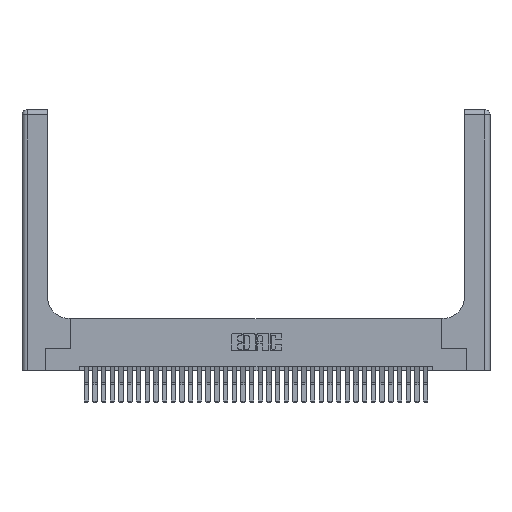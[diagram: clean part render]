
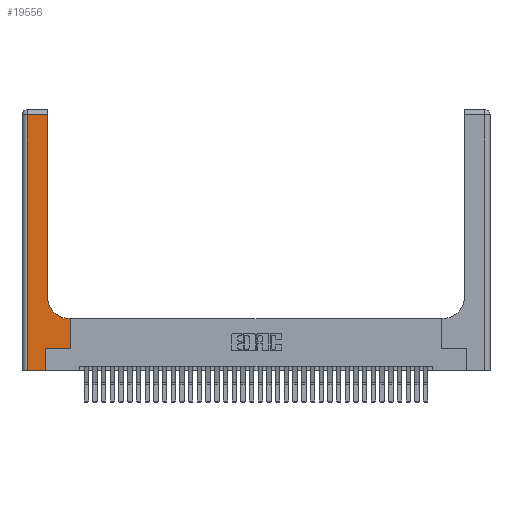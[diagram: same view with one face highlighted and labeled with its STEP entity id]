
A CAD part, top view. The second image highlights one B-rep face of the part: STEP entity #19556.
In plain terms, the highlighted planar face has unit normal (0, 0, 1).
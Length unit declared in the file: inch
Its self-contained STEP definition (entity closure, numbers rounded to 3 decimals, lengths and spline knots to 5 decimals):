
#221 = ORIENTED_EDGE ( 'NONE', *, *, #7504, .T. ) ;
#449 = DIRECTION ( 'NONE',  ( 1., 0., 0. ) ) ;
#683 = CARTESIAN_POINT ( 'NONE',  ( 0.5585, 0.25, 0.37 ) ) ;
#2005 = CARTESIAN_POINT ( 'NONE',  ( 0., 3., 0.37 ) ) ;
#2176 = ORIENTED_EDGE ( 'NONE', *, *, #9632, .T. ) ;
#2762 = CARTESIAN_POINT ( 'NONE',  ( 0., 2.94, 0.37 ) ) ;
#2857 = CARTESIAN_POINT ( 'NONE',  ( 0.2915, 0.6, 0.37 ) ) ;
#3098 = VECTOR ( 'NONE', #32187, 39.37008 ) ;
#3341 = EDGE_CURVE ( 'NONE', #21433, #3761, #20423, .T. ) ;
#3761 = VERTEX_POINT ( 'NONE', #10669 ) ;
#4089 = LINE ( 'NONE', #33217, #33562 ) ;
#4102 = CARTESIAN_POINT ( 'NONE',  ( 0.2915, 0.85, 0.37 ) ) ;
#4338 = VERTEX_POINT ( 'NONE', #13151 ) ;
#5379 = DIRECTION ( 'NONE',  ( 0., -1., 0. ) ) ;
#5756 = DIRECTION ( 'NONE',  ( -1., 0., 0. ) ) ;
#6155 = ORIENTED_EDGE ( 'NONE', *, *, #3341, .T. ) ;
#6185 = ORIENTED_EDGE ( 'NONE', *, *, #36779, .T. ) ;
#6360 = FACE_OUTER_BOUND ( 'NONE', #36173, .T. ) ;
#6371 = CARTESIAN_POINT ( 'NONE',  ( 0.5415, 0.85, 0.37 ) ) ;
#6408 = ORIENTED_EDGE ( 'NONE', *, *, #29271, .T. ) ;
#6674 = ORIENTED_EDGE ( 'NONE', *, *, #33674, .T. ) ;
#6999 = CARTESIAN_POINT ( 'NONE',  ( 0.269, 0.25, 0.37 ) ) ;
#7504 = EDGE_CURVE ( 'NONE', #4338, #23050, #27971, .T. ) ;
#9198 = AXIS2_PLACEMENT_3D ( 'NONE', #6371, #26375, #9304 ) ;
#9304 = DIRECTION ( 'NONE',  ( 1., 0., 0. ) ) ;
#9632 = EDGE_CURVE ( 'NONE', #3761, #18766, #4089, .T. ) ;
#9844 = ORIENTED_EDGE ( 'NONE', *, *, #30246, .T. ) ;
#10159 = CARTESIAN_POINT ( 'NONE',  ( 0.5585, 0.25, 0.37 ) ) ;
#10302 = ORIENTED_EDGE ( 'NONE', *, *, #11343, .T. ) ;
#10669 = CARTESIAN_POINT ( 'NONE',  ( 0.269, 0., 0.37 ) ) ;
#10811 = VERTEX_POINT ( 'NONE', #10159 ) ;
#10813 = LINE ( 'NONE', #683, #3098 ) ;
#10873 = DIRECTION ( 'NONE',  ( 1., 0., 0. ) ) ;
#11343 = EDGE_CURVE ( 'NONE', #16716, #4338, #24613, .T. ) ;
#11537 = EDGE_CURVE ( 'NONE', #18766, #10811, #25030, .T. ) ;
#12807 = VECTOR ( 'NONE', #17320, 39.37008 ) ;
#13108 = LINE ( 'NONE', #2857, #27350 ) ;
#13151 = CARTESIAN_POINT ( 'NONE',  ( 0.2915, 2.94, 0.37 ) ) ;
#13651 = DIRECTION ( 'NONE',  ( -1., 0., 0. ) ) ;
#14841 = ORIENTED_EDGE ( 'NONE', *, *, #11537, .T. ) ;
#16716 = VERTEX_POINT ( 'NONE', #4102 ) ;
#17320 = DIRECTION ( 'NONE',  ( -1., 0., 0. ) ) ;
#18687 = CARTESIAN_POINT ( 'NONE',  ( 0.2915, 3., 0.37 ) ) ;
#18766 = VERTEX_POINT ( 'NONE', #6999 ) ;
#19538 = VECTOR ( 'NONE', #449, 39.37008 ) ;
#19556 = ADVANCED_FACE ( 'NONE', ( #6360 ), #27824, .F. ) ;
#20423 = LINE ( 'NONE', #29023, #19538 ) ;
#21433 = VERTEX_POINT ( 'NONE', #22025 ) ;
#22025 = CARTESIAN_POINT ( 'NONE',  ( 0.06, 0., 0.37 ) ) ;
#22504 = VERTEX_POINT ( 'NONE', #29493 ) ;
#23050 = VERTEX_POINT ( 'NONE', #29092 ) ;
#23387 = AXIS2_PLACEMENT_3D ( 'NONE', #2005, #30648, #13651 ) ;
#24613 = LINE ( 'NONE', #18687, #30368 ) ;
#25030 = LINE ( 'NONE', #25067, #33425 ) ;
#25067 = CARTESIAN_POINT ( 'NONE',  ( 0.269, 0.25, 0.37 ) ) ;
#25405 = CARTESIAN_POINT ( 'NONE',  ( 0.06, 3., 0.37 ) ) ;
#26375 = DIRECTION ( 'NONE',  ( 0., 0., -1. ) ) ;
#27193 = DIRECTION ( 'NONE',  ( 0., 1., 0. ) ) ;
#27350 = VECTOR ( 'NONE', #5756, 39.37008 ) ;
#27824 = PLANE ( 'NONE',  #23387 ) ;
#27971 = LINE ( 'NONE', #2762, #12807 ) ;
#28368 = CARTESIAN_POINT ( 'NONE',  ( 0.5415, 0.6, 0.37 ) ) ;
#28443 = VECTOR ( 'NONE', #5379, 39.37008 ) ;
#29023 = CARTESIAN_POINT ( 'NONE',  ( 0., 0., 0.37 ) ) ;
#29092 = CARTESIAN_POINT ( 'NONE',  ( 0.06, 2.94, 0.37 ) ) ;
#29271 = EDGE_CURVE ( 'NONE', #32487, #16716, #35285, .T. ) ;
#29493 = CARTESIAN_POINT ( 'NONE',  ( 0.5585, 0.6, 0.37 ) ) ;
#30246 = EDGE_CURVE ( 'NONE', #10811, #22504, #10813, .T. ) ;
#30368 = VECTOR ( 'NONE', #27193, 39.37008 ) ;
#30648 = DIRECTION ( 'NONE',  ( 0., 0., -1. ) ) ;
#32187 = DIRECTION ( 'NONE',  ( 0., 1., 0. ) ) ;
#32487 = VERTEX_POINT ( 'NONE', #28368 ) ;
#33217 = CARTESIAN_POINT ( 'NONE',  ( 0.269, 0., 0.37 ) ) ;
#33425 = VECTOR ( 'NONE', #10873, 39.37008 ) ;
#33562 = VECTOR ( 'NONE', #33583, 39.37008 ) ;
#33583 = DIRECTION ( 'NONE',  ( 0., 1., 0. ) ) ;
#33674 = EDGE_CURVE ( 'NONE', #22504, #32487, #13108, .T. ) ;
#35285 = CIRCLE ( 'NONE', #9198, 0.25 ) ;
#36173 = EDGE_LOOP ( 'NONE', ( #10302, #221, #6185, #6155, #2176, #14841, #9844, #6674, #6408 ) ) ;
#36767 = LINE ( 'NONE', #25405, #28443 ) ;
#36779 = EDGE_CURVE ( 'NONE', #23050, #21433, #36767, .T. ) ;
